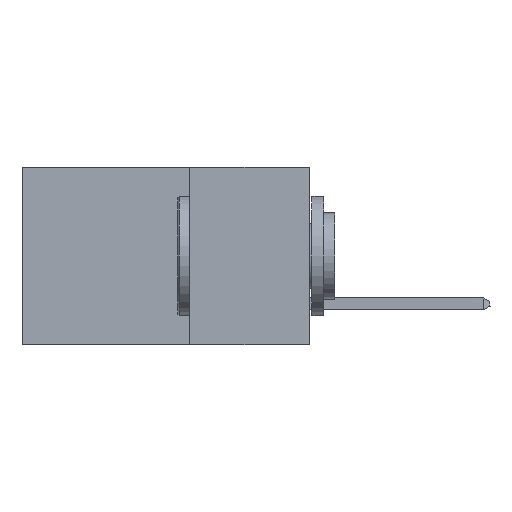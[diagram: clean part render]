
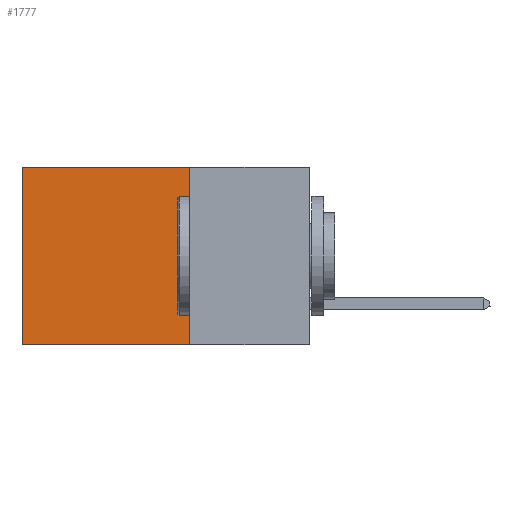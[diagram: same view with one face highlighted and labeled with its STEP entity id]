
A CAD part, left-side view. The second image highlights one B-rep face of the part: STEP entity #1777.
In plain terms, the highlighted planar face has unit normal (-1, 0, 0).
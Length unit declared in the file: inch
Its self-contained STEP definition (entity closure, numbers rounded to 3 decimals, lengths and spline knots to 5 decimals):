
#558 = LINE ( 'NONE', #5188, #13610 ) ;
#780 = EDGE_LOOP ( 'NONE', ( #6407, #17754, #12867, #6100 ) ) ;
#1777 = ADVANCED_FACE ( 'NONE', ( #27310 ), #41240, .F. ) ;
#2214 = VECTOR ( 'NONE', #20686, 39.37008 ) ;
#4638 = CARTESIAN_POINT ( 'NONE',  ( 0.2875, 0.25, -0.37 ) ) ;
#4845 = LINE ( 'NONE', #9265, #32145 ) ;
#5188 = CARTESIAN_POINT ( 'NONE',  ( 0.2875, 0.6, 0. ) ) ;
#5963 = CARTESIAN_POINT ( 'NONE',  ( 0.2875, 0.25, 0. ) ) ;
#6100 = ORIENTED_EDGE ( 'NONE', *, *, #21615, .T. ) ;
#6407 = ORIENTED_EDGE ( 'NONE', *, *, #10733, .T. ) ;
#9265 = CARTESIAN_POINT ( 'NONE',  ( 0.2875, 0.25, -0.37 ) ) ;
#10733 = EDGE_CURVE ( 'NONE', #39802, #25239, #558, .T. ) ;
#12867 = ORIENTED_EDGE ( 'NONE', *, *, #28760, .F. ) ;
#13610 = VECTOR ( 'NONE', #45558, 39.37008 ) ;
#16171 = EDGE_CURVE ( 'NONE', #21652, #25239, #4845, .T. ) ;
#17754 = ORIENTED_EDGE ( 'NONE', *, *, #16171, .F. ) ;
#19701 = DIRECTION ( 'NONE',  ( 1., 0., 0. ) ) ;
#20671 = VECTOR ( 'NONE', #27627, 39.37008 ) ;
#20686 = DIRECTION ( 'NONE',  ( 0., 0., -1. ) ) ;
#21615 = EDGE_CURVE ( 'NONE', #41068, #39802, #46327, .T. ) ;
#21652 = VERTEX_POINT ( 'NONE', #4638 ) ;
#21997 = LINE ( 'NONE', #5963, #2214 ) ;
#23563 = DIRECTION ( 'NONE',  ( 0., 1., 0. ) ) ;
#25239 = VERTEX_POINT ( 'NONE', #40121 ) ;
#27051 = DIRECTION ( 'NONE',  ( 0., 0., -1. ) ) ;
#27310 = FACE_OUTER_BOUND ( 'NONE', #780, .T. ) ;
#27627 = DIRECTION ( 'NONE',  ( 0., 1., 0. ) ) ;
#28354 = CARTESIAN_POINT ( 'NONE',  ( 0.2875, 0.25, 0. ) ) ;
#28760 = EDGE_CURVE ( 'NONE', #41068, #21652, #21997, .T. ) ;
#30867 = CARTESIAN_POINT ( 'NONE',  ( 0.2875, 0.25, 0. ) ) ;
#32145 = VECTOR ( 'NONE', #23563, 39.37008 ) ;
#39802 = VERTEX_POINT ( 'NONE', #44627 ) ;
#40121 = CARTESIAN_POINT ( 'NONE',  ( 0.2875, 0.6, -0.37 ) ) ;
#40606 = AXIS2_PLACEMENT_3D ( 'NONE', #30867, #19701, #27051 ) ;
#41068 = VERTEX_POINT ( 'NONE', #42160 ) ;
#41240 = PLANE ( 'NONE',  #40606 ) ;
#42160 = CARTESIAN_POINT ( 'NONE',  ( 0.2875, 0.25, 0. ) ) ;
#44627 = CARTESIAN_POINT ( 'NONE',  ( 0.2875, 0.6, 0. ) ) ;
#45558 = DIRECTION ( 'NONE',  ( 0., 0., -1. ) ) ;
#46327 = LINE ( 'NONE', #28354, #20671 ) ;
